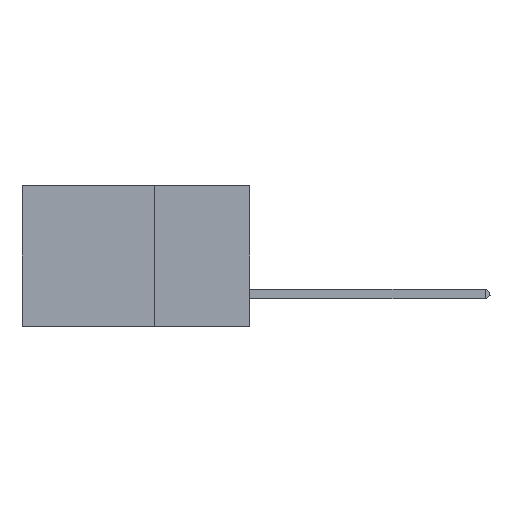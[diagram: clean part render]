
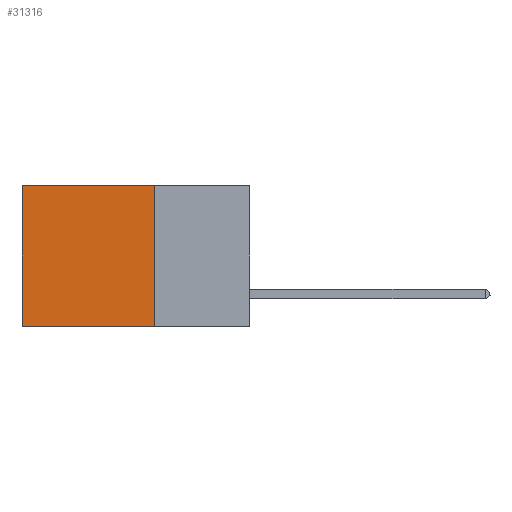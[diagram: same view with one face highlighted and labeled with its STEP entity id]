
A CAD part, left-side view. The second image highlights one B-rep face of the part: STEP entity #31316.
In plain terms, the highlighted planar face has unit normal (-1, 0, 0).
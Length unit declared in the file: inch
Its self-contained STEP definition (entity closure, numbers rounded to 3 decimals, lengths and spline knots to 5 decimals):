
#794 = FACE_OUTER_BOUND ( 'NONE', #31180, .T. ) ;
#1929 = CARTESIAN_POINT ( 'NONE',  ( 0.2875, 0.6, 0. ) ) ;
#4670 = VERTEX_POINT ( 'NONE', #5602 ) ;
#4780 = DIRECTION ( 'NONE',  ( 0., 0., -1. ) ) ;
#5602 = CARTESIAN_POINT ( 'NONE',  ( 0.2875, 0.25, -0.37 ) ) ;
#6878 = CARTESIAN_POINT ( 'NONE',  ( 0.2875, 0.25, 0. ) ) ;
#8865 = AXIS2_PLACEMENT_3D ( 'NONE', #6878, #25542, #33274 ) ;
#9018 = DIRECTION ( 'NONE',  ( 0., 0., -1. ) ) ;
#9416 = ORIENTED_EDGE ( 'NONE', *, *, #26053, .T. ) ;
#9439 = DIRECTION ( 'NONE',  ( 0., 1., 0. ) ) ;
#9795 = VERTEX_POINT ( 'NONE', #1929 ) ;
#10553 = VERTEX_POINT ( 'NONE', #22454 ) ;
#11348 = ORIENTED_EDGE ( 'NONE', *, *, #17173, .T. ) ;
#13465 = LINE ( 'NONE', #28202, #18827 ) ;
#14100 = LINE ( 'NONE', #32225, #21894 ) ;
#15065 = VERTEX_POINT ( 'NONE', #20021 ) ;
#15175 = VECTOR ( 'NONE', #9439, 39.37008 ) ;
#17173 = EDGE_CURVE ( 'NONE', #15065, #9795, #14100, .T. ) ;
#17632 = LINE ( 'NONE', #22515, #15175 ) ;
#18827 = VECTOR ( 'NONE', #4780, 39.37008 ) ;
#20021 = CARTESIAN_POINT ( 'NONE',  ( 0.2875, 0.25, 0. ) ) ;
#21872 = DIRECTION ( 'NONE',  ( 0., 1., 0. ) ) ;
#21894 = VECTOR ( 'NONE', #21872, 39.37008 ) ;
#22454 = CARTESIAN_POINT ( 'NONE',  ( 0.2875, 0.6, -0.37 ) ) ;
#22515 = CARTESIAN_POINT ( 'NONE',  ( 0.2875, 0.25, -0.37 ) ) ;
#23752 = EDGE_CURVE ( 'NONE', #15065, #4670, #30428, .T. ) ;
#25324 = EDGE_CURVE ( 'NONE', #4670, #10553, #17632, .T. ) ;
#25542 = DIRECTION ( 'NONE',  ( 1., 0., 0. ) ) ;
#25869 = VECTOR ( 'NONE', #9018, 39.37008 ) ;
#26053 = EDGE_CURVE ( 'NONE', #9795, #10553, #13465, .T. ) ;
#26129 = ORIENTED_EDGE ( 'NONE', *, *, #25324, .F. ) ;
#27702 = CARTESIAN_POINT ( 'NONE',  ( 0.2875, 0.25, 0. ) ) ;
#27984 = PLANE ( 'NONE',  #8865 ) ;
#28202 = CARTESIAN_POINT ( 'NONE',  ( 0.2875, 0.6, 0. ) ) ;
#30203 = ORIENTED_EDGE ( 'NONE', *, *, #23752, .F. ) ;
#30428 = LINE ( 'NONE', #27702, #25869 ) ;
#31180 = EDGE_LOOP ( 'NONE', ( #9416, #26129, #30203, #11348 ) ) ;
#31316 = ADVANCED_FACE ( 'NONE', ( #794 ), #27984, .F. ) ;
#32225 = CARTESIAN_POINT ( 'NONE',  ( 0.2875, 0.25, 0. ) ) ;
#33274 = DIRECTION ( 'NONE',  ( 0., 0., -1. ) ) ;
